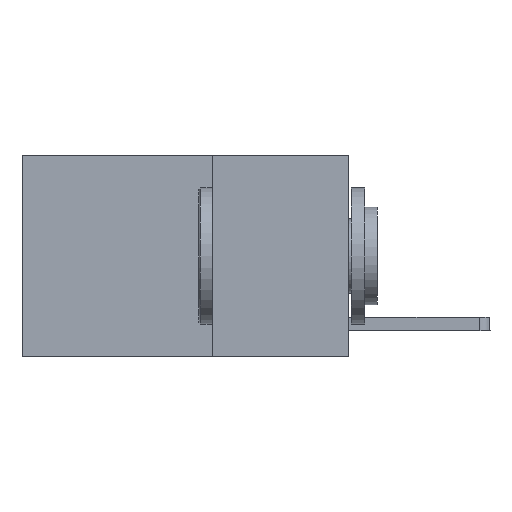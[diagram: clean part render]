
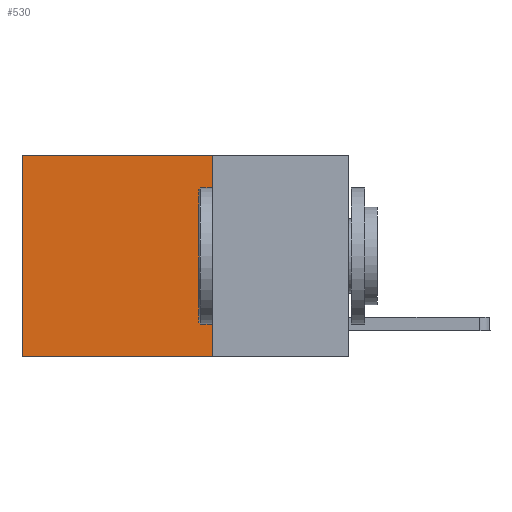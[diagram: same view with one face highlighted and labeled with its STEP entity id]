
A CAD part, left-side view. The second image highlights one B-rep face of the part: STEP entity #530.
In plain terms, the highlighted planar face has unit normal (-1, 0, 0).
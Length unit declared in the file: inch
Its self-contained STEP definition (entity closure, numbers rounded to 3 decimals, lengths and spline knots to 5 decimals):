
#115 = EDGE_CURVE ( 'NONE', #6942, #5125, #3228, .T. ) ;
#350 = CARTESIAN_POINT ( 'NONE',  ( 0.2625, 0.6, -0.37 ) ) ;
#530 = ADVANCED_FACE ( 'NONE', ( #1631 ), #7146, .F. ) ;
#956 = CARTESIAN_POINT ( 'NONE',  ( 0.2625, 0.25, 0. ) ) ;
#1255 = DIRECTION ( 'NONE',  ( 0., 0., -1. ) ) ;
#1631 = FACE_OUTER_BOUND ( 'NONE', #3692, .T. ) ;
#1993 = VERTEX_POINT ( 'NONE', #350 ) ;
#2440 = DIRECTION ( 'NONE',  ( 0., 0., -1. ) ) ;
#2631 = ORIENTED_EDGE ( 'NONE', *, *, #5994, .T. ) ;
#2651 = VERTEX_POINT ( 'NONE', #4820 ) ;
#2713 = CARTESIAN_POINT ( 'NONE',  ( 0.2625, 0.25, 0. ) ) ;
#2858 = ORIENTED_EDGE ( 'NONE', *, *, #115, .F. ) ;
#3228 = LINE ( 'NONE', #9806, #3687 ) ;
#3687 = VECTOR ( 'NONE', #2440, 39.37008 ) ;
#3692 = EDGE_LOOP ( 'NONE', ( #2631, #4064, #2858, #4874 ) ) ;
#3886 = CARTESIAN_POINT ( 'NONE',  ( 0.2625, 0.25, -0.37 ) ) ;
#3980 = LINE ( 'NONE', #8934, #7710 ) ;
#4064 = ORIENTED_EDGE ( 'NONE', *, *, #9315, .F. ) ;
#4169 = LINE ( 'NONE', #2713, #5441 ) ;
#4820 = CARTESIAN_POINT ( 'NONE',  ( 0.2625, 0.6, 0. ) ) ;
#4874 = ORIENTED_EDGE ( 'NONE', *, *, #7635, .T. ) ;
#5125 = VERTEX_POINT ( 'NONE', #3886 ) ;
#5441 = VECTOR ( 'NONE', #9289, 39.37008 ) ;
#5703 = DIRECTION ( 'NONE',  ( 0., 1., 0. ) ) ;
#5907 = VECTOR ( 'NONE', #1255, 39.37008 ) ;
#5994 = EDGE_CURVE ( 'NONE', #2651, #1993, #7908, .T. ) ;
#6268 = CARTESIAN_POINT ( 'NONE',  ( 0.2625, 0.6, 0. ) ) ;
#6942 = VERTEX_POINT ( 'NONE', #9604 ) ;
#7146 = PLANE ( 'NONE',  #7620 ) ;
#7620 = AXIS2_PLACEMENT_3D ( 'NONE', #956, #8322, #10446 ) ;
#7635 = EDGE_CURVE ( 'NONE', #6942, #2651, #4169, .T. ) ;
#7710 = VECTOR ( 'NONE', #5703, 39.37008 ) ;
#7908 = LINE ( 'NONE', #6268, #5907 ) ;
#8322 = DIRECTION ( 'NONE',  ( 1., 0., 0. ) ) ;
#8934 = CARTESIAN_POINT ( 'NONE',  ( 0.2625, 0.25, -0.37 ) ) ;
#9289 = DIRECTION ( 'NONE',  ( 0., 1., 0. ) ) ;
#9315 = EDGE_CURVE ( 'NONE', #5125, #1993, #3980, .T. ) ;
#9604 = CARTESIAN_POINT ( 'NONE',  ( 0.2625, 0.25, 0. ) ) ;
#9806 = CARTESIAN_POINT ( 'NONE',  ( 0.2625, 0.25, 0. ) ) ;
#10446 = DIRECTION ( 'NONE',  ( 0., 0., -1. ) ) ;
